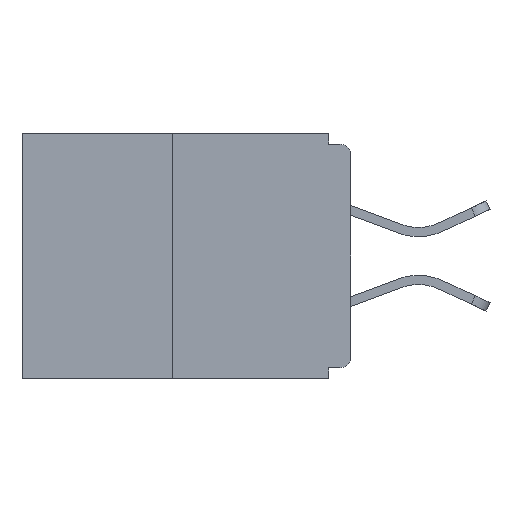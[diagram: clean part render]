
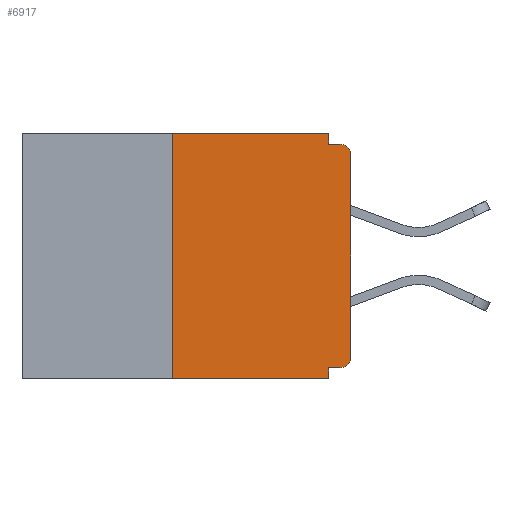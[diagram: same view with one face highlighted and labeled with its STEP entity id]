
A CAD part, left-side view. The second image highlights one B-rep face of the part: STEP entity #6917.
In plain terms, the highlighted planar face has unit normal (-1, 0, 0).
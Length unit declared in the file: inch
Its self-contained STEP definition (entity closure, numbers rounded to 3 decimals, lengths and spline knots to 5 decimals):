
#205 = CARTESIAN_POINT ( 'NONE',  ( 0., 0.031, 0. ) ) ;
#249 = CARTESIAN_POINT ( 'NONE',  ( 0., 0.015, -0.313 ) ) ;
#293 = EDGE_CURVE ( 'NONE', #711, #15274, #9325, .T. ) ;
#391 = VECTOR ( 'NONE', #7533, 39.37008 ) ;
#486 = DIRECTION ( 'NONE',  ( 0., -1., 0. ) ) ;
#711 = VERTEX_POINT ( 'NONE', #205 ) ;
#809 = CARTESIAN_POINT ( 'NONE',  ( 0., 0.031, -0.328 ) ) ;
#851 = ORIENTED_EDGE ( 'NONE', *, *, #1541, .F. ) ;
#1088 = EDGE_CURVE ( 'NONE', #12705, #13689, #15022, .T. ) ;
#1236 = CARTESIAN_POINT ( 'NONE',  ( 0., 0., -0.328 ) ) ;
#1429 = LINE ( 'NONE', #7071, #8954 ) ;
#1523 = CARTESIAN_POINT ( 'NONE',  ( 0., 0., -0.03 ) ) ;
#1541 = EDGE_CURVE ( 'NONE', #12318, #711, #8304, .T. ) ;
#2048 = AXIS2_PLACEMENT_3D ( 'NONE', #10990, #14777, #16002 ) ;
#2223 = LINE ( 'NONE', #12228, #13074 ) ;
#2411 = ORIENTED_EDGE ( 'NONE', *, *, #12762, .T. ) ;
#2800 = LINE ( 'NONE', #10728, #10897 ) ;
#3155 = FACE_OUTER_BOUND ( 'NONE', #10960, .T. ) ;
#3413 = VECTOR ( 'NONE', #9636, 39.37008 ) ;
#3798 = VECTOR ( 'NONE', #8867, 39.37008 ) ;
#3902 = CARTESIAN_POINT ( 'NONE',  ( 0., 0.031, -0.015 ) ) ;
#4073 = DIRECTION ( 'NONE',  ( 0., 0., -1. ) ) ;
#4092 = EDGE_CURVE ( 'NONE', #8850, #12493, #6221, .T. ) ;
#4317 = CARTESIAN_POINT ( 'NONE',  ( 0., 0.031, -0.343 ) ) ;
#4402 = EDGE_CURVE ( 'NONE', #6978, #12955, #13890, .T. ) ;
#4476 = DIRECTION ( 'NONE',  ( 0., 0., 1. ) ) ;
#4656 = AXIS2_PLACEMENT_3D ( 'NONE', #249, #9080, #4073 ) ;
#5186 = CARTESIAN_POINT ( 'NONE',  ( 0., 0.015, -0.328 ) ) ;
#5270 = EDGE_CURVE ( 'NONE', #15274, #12955, #2223, .T. ) ;
#5456 = ORIENTED_EDGE ( 'NONE', *, *, #4092, .T. ) ;
#5954 = EDGE_CURVE ( 'NONE', #8850, #12705, #10492, .T. ) ;
#6068 = PLANE ( 'NONE',  #2048 ) ;
#6221 = CIRCLE ( 'NONE', #4656, 0.015 ) ;
#6543 = ORIENTED_EDGE ( 'NONE', *, *, #5954, .F. ) ;
#6917 = ADVANCED_FACE ( 'NONE', ( #3155 ), #6068, .F. ) ;
#6978 = VERTEX_POINT ( 'NONE', #1523 ) ;
#6988 = AXIS2_PLACEMENT_3D ( 'NONE', #14602, #8288, #9545 ) ;
#7071 = CARTESIAN_POINT ( 'NONE',  ( 0., 0., 0. ) ) ;
#7123 = LINE ( 'NONE', #13254, #14396 ) ;
#7205 = ORIENTED_EDGE ( 'NONE', *, *, #1088, .F. ) ;
#7533 = DIRECTION ( 'NONE',  ( 0., 0., -1. ) ) ;
#8288 = DIRECTION ( 'NONE',  ( -1., 0., 0. ) ) ;
#8304 = LINE ( 'NONE', #15736, #14590 ) ;
#8384 = CARTESIAN_POINT ( 'NONE',  ( 0., 0.031, 0. ) ) ;
#8509 = DIRECTION ( 'NONE',  ( 0., -1., 0. ) ) ;
#8850 = VERTEX_POINT ( 'NONE', #5186 ) ;
#8867 = DIRECTION ( 'NONE',  ( 0., 1., 0. ) ) ;
#8954 = VECTOR ( 'NONE', #4476, 39.37008 ) ;
#9080 = DIRECTION ( 'NONE',  ( -1., 0., 0. ) ) ;
#9325 = LINE ( 'NONE', #8384, #3413 ) ;
#9545 = DIRECTION ( 'NONE',  ( 0., 0., -1. ) ) ;
#9636 = DIRECTION ( 'NONE',  ( 0., 0., -1. ) ) ;
#9714 = CARTESIAN_POINT ( 'NONE',  ( 0., 0.25, 0. ) ) ;
#10351 = ORIENTED_EDGE ( 'NONE', *, *, #4402, .T. ) ;
#10492 = LINE ( 'NONE', #1236, #3798 ) ;
#10594 = ORIENTED_EDGE ( 'NONE', *, *, #13461, .T. ) ;
#10728 = CARTESIAN_POINT ( 'NONE',  ( 0., 0.46, -0.343 ) ) ;
#10897 = VECTOR ( 'NONE', #14629, 39.37008 ) ;
#10960 = EDGE_LOOP ( 'NONE', ( #851, #14955, #10594, #7205, #6543, #5456, #2411, #10351, #12996, #14935 ) ) ;
#10990 = CARTESIAN_POINT ( 'NONE',  ( 0., 0.46, 0. ) ) ;
#12228 = CARTESIAN_POINT ( 'NONE',  ( 0., 0., -0.015 ) ) ;
#12318 = VERTEX_POINT ( 'NONE', #9714 ) ;
#12446 = CARTESIAN_POINT ( 'NONE',  ( 0., 0.015, -0.015 ) ) ;
#12493 = VERTEX_POINT ( 'NONE', #14242 ) ;
#12597 = CARTESIAN_POINT ( 'NONE',  ( 0., 0.031, -0.343 ) ) ;
#12705 = VERTEX_POINT ( 'NONE', #809 ) ;
#12762 = EDGE_CURVE ( 'NONE', #12493, #6978, #1429, .T. ) ;
#12955 = VERTEX_POINT ( 'NONE', #12446 ) ;
#12996 = ORIENTED_EDGE ( 'NONE', *, *, #5270, .F. ) ;
#13074 = VECTOR ( 'NONE', #8509, 39.37008 ) ;
#13254 = CARTESIAN_POINT ( 'NONE',  ( 0., 0.25, 0. ) ) ;
#13346 = CARTESIAN_POINT ( 'NONE',  ( 0., 0.25, -0.343 ) ) ;
#13461 = EDGE_CURVE ( 'NONE', #15699, #13689, #2800, .T. ) ;
#13689 = VERTEX_POINT ( 'NONE', #4317 ) ;
#13890 = CIRCLE ( 'NONE', #6988, 0.015 ) ;
#14138 = EDGE_CURVE ( 'NONE', #15699, #12318, #7123, .T. ) ;
#14242 = CARTESIAN_POINT ( 'NONE',  ( 0., 0., -0.313 ) ) ;
#14396 = VECTOR ( 'NONE', #16024, 39.37008 ) ;
#14590 = VECTOR ( 'NONE', #486, 39.37008 ) ;
#14602 = CARTESIAN_POINT ( 'NONE',  ( 0., 0.015, -0.03 ) ) ;
#14629 = DIRECTION ( 'NONE',  ( 0., -1., 0. ) ) ;
#14777 = DIRECTION ( 'NONE',  ( 1., 0., 0. ) ) ;
#14935 = ORIENTED_EDGE ( 'NONE', *, *, #293, .F. ) ;
#14955 = ORIENTED_EDGE ( 'NONE', *, *, #14138, .F. ) ;
#15022 = LINE ( 'NONE', #12597, #391 ) ;
#15274 = VERTEX_POINT ( 'NONE', #3902 ) ;
#15699 = VERTEX_POINT ( 'NONE', #13346 ) ;
#15736 = CARTESIAN_POINT ( 'NONE',  ( 0., 0.46, 0. ) ) ;
#16002 = DIRECTION ( 'NONE',  ( 0., 0., -1. ) ) ;
#16024 = DIRECTION ( 'NONE',  ( 0., 0., 1. ) ) ;
